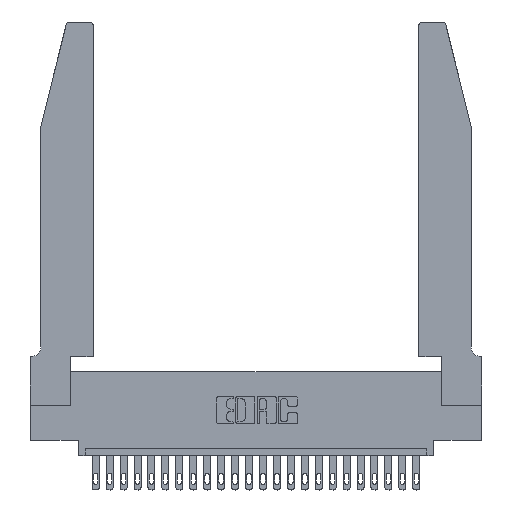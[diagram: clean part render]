
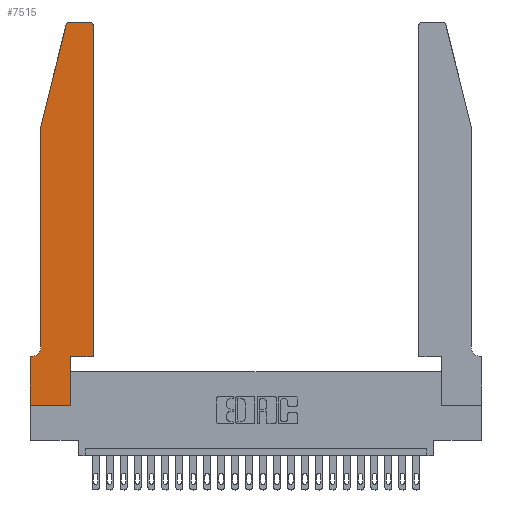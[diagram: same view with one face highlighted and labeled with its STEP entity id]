
A CAD part, top view. The second image highlights one B-rep face of the part: STEP entity #7515.
In plain terms, the highlighted planar face has unit normal (0, 0, 1).
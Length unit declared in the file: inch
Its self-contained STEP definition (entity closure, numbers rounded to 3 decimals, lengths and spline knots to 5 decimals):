
#127 = CARTESIAN_POINT ( 'NONE',  ( 0.4205, 2.72, 0.37 ) ) ;
#389 = EDGE_CURVE ( 'NONE', #9436, #13447, #5412, .T. ) ;
#818 = CIRCLE ( 'NONE', #23054, 0.03 ) ;
#1030 = ORIENTED_EDGE ( 'NONE', *, *, #25225, .T. ) ;
#1172 = VECTOR ( 'NONE', #23030, 39.37008 ) ;
#1270 = EDGE_CURVE ( 'NONE', #1736, #9630, #20716, .T. ) ;
#1447 = VERTEX_POINT ( 'NONE', #6920 ) ;
#1736 = VERTEX_POINT ( 'NONE', #10406 ) ;
#1821 = LINE ( 'NONE', #17190, #12811 ) ;
#1970 = LINE ( 'NONE', #6442, #4681 ) ;
#3420 = DIRECTION ( 'NONE',  ( -0.239, -0.971, 0. ) ) ;
#3540 = CARTESIAN_POINT ( 'NONE',  ( 0.0055, 0.35, 0.37 ) ) ;
#3748 = EDGE_CURVE ( 'NONE', #7606, #24682, #1970, .T. ) ;
#4598 = AXIS2_PLACEMENT_3D ( 'NONE', #24055, #18352, #10389 ) ;
#4681 = VECTOR ( 'NONE', #24144, 39.37008 ) ;
#4891 = VECTOR ( 'NONE', #7339, 39.37008 ) ;
#5059 = EDGE_CURVE ( 'NONE', #19186, #7874, #20243, .T. ) ;
#5412 = LINE ( 'NONE', #5845, #6629 ) ;
#5591 = VECTOR ( 'NONE', #6089, 39.37008 ) ;
#5668 = EDGE_CURVE ( 'NONE', #20133, #16107, #15006, .T. ) ;
#5845 = CARTESIAN_POINT ( 'NONE',  ( 0., 0., 0.37 ) ) ;
#5859 = LINE ( 'NONE', #7957, #5591 ) ;
#6089 = DIRECTION ( 'NONE',  ( 1., 0., 0. ) ) ;
#6243 = CARTESIAN_POINT ( 'NONE',  ( 0., 0., 0.37 ) ) ;
#6438 = CARTESIAN_POINT ( 'NONE',  ( 0.0055, 0.42, 0.37 ) ) ;
#6442 = CARTESIAN_POINT ( 'NONE',  ( 0.0755, 0.35, 0.37 ) ) ;
#6629 = VECTOR ( 'NONE', #24447, 39.37008 ) ;
#6920 = CARTESIAN_POINT ( 'NONE',  ( 0.25487, 2.72718, 0.37 ) ) ;
#6973 = ORIENTED_EDGE ( 'NONE', *, *, #389, .T. ) ;
#7339 = DIRECTION ( 'NONE',  ( 0., -1., 0. ) ) ;
#7515 = ADVANCED_FACE ( 'NONE', ( #13073 ), #14794, .T. ) ;
#7606 = VERTEX_POINT ( 'NONE', #3540 ) ;
#7842 = CARTESIAN_POINT ( 'NONE',  ( 0.0755, 2., 0.37 ) ) ;
#7874 = VERTEX_POINT ( 'NONE', #24676 ) ;
#7957 = CARTESIAN_POINT ( 'NONE',  ( 0.4505, 0.35, 0.37 ) ) ;
#8067 = CIRCLE ( 'NONE', #22481, 0.07 ) ;
#8319 = CARTESIAN_POINT ( 'NONE',  ( 0.2865, 0.35, 0.37 ) ) ;
#9266 = ORIENTED_EDGE ( 'NONE', *, *, #5059, .T. ) ;
#9436 = VERTEX_POINT ( 'NONE', #6243 ) ;
#9630 = VERTEX_POINT ( 'NONE', #24631 ) ;
#9788 = ORIENTED_EDGE ( 'NONE', *, *, #24271, .T. ) ;
#10228 = ORIENTED_EDGE ( 'NONE', *, *, #13742, .T. ) ;
#10389 = DIRECTION ( 'NONE',  ( 1., 0., 0. ) ) ;
#10406 = CARTESIAN_POINT ( 'NONE',  ( 0.4505, 0.35, 0.37 ) ) ;
#10645 = DIRECTION ( 'NONE',  ( -1., 0., 0. ) ) ;
#10805 = EDGE_CURVE ( 'NONE', #15105, #1736, #5859, .T. ) ;
#11049 = CARTESIAN_POINT ( 'NONE',  ( 0.0755, 2., 0.37 ) ) ;
#11690 = DIRECTION ( 'NONE',  ( 0., 0., 1. ) ) ;
#12210 = ORIENTED_EDGE ( 'NONE', *, *, #3748, .T. ) ;
#12769 = LINE ( 'NONE', #19137, #22568 ) ;
#12811 = VECTOR ( 'NONE', #3420, 39.37008 ) ;
#13007 = ORIENTED_EDGE ( 'NONE', *, *, #24357, .T. ) ;
#13073 = FACE_OUTER_BOUND ( 'NONE', #15531, .T. ) ;
#13197 = CARTESIAN_POINT ( 'NONE',  ( 0., 0.35, 0.37 ) ) ;
#13323 = CARTESIAN_POINT ( 'NONE',  ( 0.4205, 2.75, 0.37 ) ) ;
#13447 = VERTEX_POINT ( 'NONE', #13571 ) ;
#13571 = CARTESIAN_POINT ( 'NONE',  ( 0.2865, 0., 0.37 ) ) ;
#13742 = EDGE_CURVE ( 'NONE', #7874, #1447, #21359, .T. ) ;
#14317 = DIRECTION ( 'NONE',  ( 0., 0., -1. ) ) ;
#14794 = PLANE ( 'NONE',  #24625 ) ;
#14896 = LINE ( 'NONE', #14985, #1172 ) ;
#14985 = CARTESIAN_POINT ( 'NONE',  ( 0.2865, 0.35, 0.37 ) ) ;
#15006 = LINE ( 'NONE', #11049, #4891 ) ;
#15105 = VERTEX_POINT ( 'NONE', #8319 ) ;
#15531 = EDGE_LOOP ( 'NONE', ( #9266, #10228, #19226, #22115, #1030, #12210, #13007, #6973, #9788, #16482, #23918, #18229 ) ) ;
#15744 = DIRECTION ( 'NONE',  ( 0., 1., 0. ) ) ;
#16107 = VERTEX_POINT ( 'NONE', #23411 ) ;
#16482 = ORIENTED_EDGE ( 'NONE', *, *, #10805, .T. ) ;
#17190 = CARTESIAN_POINT ( 'NONE',  ( 0.0755, 2., 0.37 ) ) ;
#17559 = CARTESIAN_POINT ( 'NONE',  ( 0.4505, 0.35, 0.37 ) ) ;
#18229 = ORIENTED_EDGE ( 'NONE', *, *, #19911, .T. ) ;
#18352 = DIRECTION ( 'NONE',  ( 0., 0., 1. ) ) ;
#19040 = EDGE_CURVE ( 'NONE', #1447, #20133, #1821, .T. ) ;
#19137 = CARTESIAN_POINT ( 'NONE',  ( 0., 0., 0.37 ) ) ;
#19186 = VERTEX_POINT ( 'NONE', #13323 ) ;
#19218 = DIRECTION ( 'NONE',  ( 0., -1., 0. ) ) ;
#19226 = ORIENTED_EDGE ( 'NONE', *, *, #19040, .T. ) ;
#19911 = EDGE_CURVE ( 'NONE', #9630, #19186, #818, .T. ) ;
#19925 = DIRECTION ( 'NONE',  ( -1., 0., 0. ) ) ;
#20133 = VERTEX_POINT ( 'NONE', #7842 ) ;
#20243 = LINE ( 'NONE', #20271, #22062 ) ;
#20271 = CARTESIAN_POINT ( 'NONE',  ( 0.2605, 2.75, 0.37 ) ) ;
#20716 = LINE ( 'NONE', #17559, #24328 ) ;
#21059 = DIRECTION ( 'NONE',  ( 0., 0., 1. ) ) ;
#21359 = CIRCLE ( 'NONE', #4598, 0.03 ) ;
#21624 = DIRECTION ( 'NONE',  ( 1., 0., 0. ) ) ;
#21811 = DIRECTION ( 'NONE',  ( 1., 0., 0. ) ) ;
#22062 = VECTOR ( 'NONE', #19925, 39.37008 ) ;
#22115 = ORIENTED_EDGE ( 'NONE', *, *, #5668, .T. ) ;
#22481 = AXIS2_PLACEMENT_3D ( 'NONE', #6438, #14317, #10645 ) ;
#22568 = VECTOR ( 'NONE', #19218, 39.37008 ) ;
#23030 = DIRECTION ( 'NONE',  ( 0., 1., 0. ) ) ;
#23054 = AXIS2_PLACEMENT_3D ( 'NONE', #127, #11690, #21624 ) ;
#23411 = CARTESIAN_POINT ( 'NONE',  ( 0.0755, 0.42, 0.37 ) ) ;
#23918 = ORIENTED_EDGE ( 'NONE', *, *, #1270, .T. ) ;
#24055 = CARTESIAN_POINT ( 'NONE',  ( 0.284, 2.72, 0.37 ) ) ;
#24144 = DIRECTION ( 'NONE',  ( -1., 0., 0. ) ) ;
#24249 = CARTESIAN_POINT ( 'NONE',  ( 0., 0.35, 0.37 ) ) ;
#24271 = EDGE_CURVE ( 'NONE', #13447, #15105, #14896, .T. ) ;
#24328 = VECTOR ( 'NONE', #15744, 39.37008 ) ;
#24357 = EDGE_CURVE ( 'NONE', #24682, #9436, #12769, .T. ) ;
#24447 = DIRECTION ( 'NONE',  ( 1., 0., 0. ) ) ;
#24625 = AXIS2_PLACEMENT_3D ( 'NONE', #13197, #21059, #21811 ) ;
#24631 = CARTESIAN_POINT ( 'NONE',  ( 0.4505, 2.72, 0.37 ) ) ;
#24676 = CARTESIAN_POINT ( 'NONE',  ( 0.284, 2.75, 0.37 ) ) ;
#24682 = VERTEX_POINT ( 'NONE', #24249 ) ;
#25225 = EDGE_CURVE ( 'NONE', #16107, #7606, #8067, .T. ) ;
